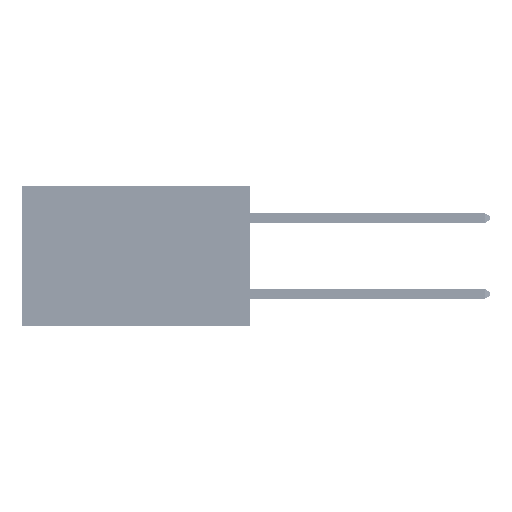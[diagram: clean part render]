
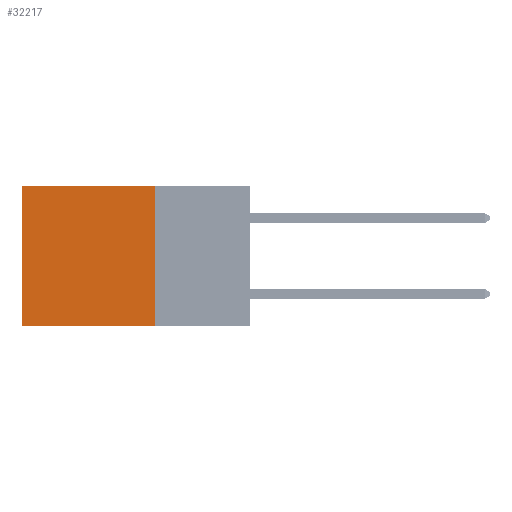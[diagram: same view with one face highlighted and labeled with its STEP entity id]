
A CAD part, left-side view. The second image highlights one B-rep face of the part: STEP entity #32217.
In plain terms, the highlighted planar face has unit normal (-1, 0, 0).
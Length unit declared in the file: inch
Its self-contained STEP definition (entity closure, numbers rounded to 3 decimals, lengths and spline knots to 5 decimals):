
#485 = DIRECTION ( 'NONE',  ( 1., 0., 0. ) ) ;
#1061 = CARTESIAN_POINT ( 'NONE',  ( 0.2875, 0.25, 0. ) ) ;
#2363 = VERTEX_POINT ( 'NONE', #25750 ) ;
#6617 = EDGE_CURVE ( 'NONE', #17309, #47645, #27019, .T. ) ;
#7223 = VECTOR ( 'NONE', #8828, 39.37008 ) ;
#8828 = DIRECTION ( 'NONE',  ( 0., 0., -1. ) ) ;
#8851 = FACE_OUTER_BOUND ( 'NONE', #42961, .T. ) ;
#9224 = CARTESIAN_POINT ( 'NONE',  ( 0.2875, 0.6, 0. ) ) ;
#10294 = ORIENTED_EDGE ( 'NONE', *, *, #19120, .T. ) ;
#11267 = PLANE ( 'NONE',  #15347 ) ;
#12152 = EDGE_CURVE ( 'NONE', #47645, #2363, #40489, .T. ) ;
#15113 = CARTESIAN_POINT ( 'NONE',  ( 0.2875, 0.25, 0. ) ) ;
#15347 = AXIS2_PLACEMENT_3D ( 'NONE', #15113, #485, #38508 ) ;
#17309 = VERTEX_POINT ( 'NONE', #34848 ) ;
#18458 = ORIENTED_EDGE ( 'NONE', *, *, #20578, .T. ) ;
#19120 = EDGE_CURVE ( 'NONE', #31198, #2363, #48873, .T. ) ;
#20578 = EDGE_CURVE ( 'NONE', #17309, #31198, #47485, .T. ) ;
#22829 = VECTOR ( 'NONE', #48923, 39.37008 ) ;
#25750 = CARTESIAN_POINT ( 'NONE',  ( 0.2875, 0.6, -0.37 ) ) ;
#27019 = LINE ( 'NONE', #1061, #7223 ) ;
#27692 = CARTESIAN_POINT ( 'NONE',  ( 0.2875, 0.25, -0.37 ) ) ;
#28824 = ORIENTED_EDGE ( 'NONE', *, *, #12152, .F. ) ;
#31198 = VERTEX_POINT ( 'NONE', #47974 ) ;
#32122 = DIRECTION ( 'NONE',  ( 0., 0., -1. ) ) ;
#32217 = ADVANCED_FACE ( 'NONE', ( #8851 ), #11267, .F. ) ;
#32689 = VECTOR ( 'NONE', #34428, 39.37008 ) ;
#34428 = DIRECTION ( 'NONE',  ( 0., 1., 0. ) ) ;
#34848 = CARTESIAN_POINT ( 'NONE',  ( 0.2875, 0.25, 0. ) ) ;
#37218 = CARTESIAN_POINT ( 'NONE',  ( 0.2875, 0.25, 0. ) ) ;
#38508 = DIRECTION ( 'NONE',  ( 0., 0., -1. ) ) ;
#38699 = VECTOR ( 'NONE', #32122, 39.37008 ) ;
#40489 = LINE ( 'NONE', #46024, #32689 ) ;
#41326 = ORIENTED_EDGE ( 'NONE', *, *, #6617, .F. ) ;
#42961 = EDGE_LOOP ( 'NONE', ( #10294, #28824, #41326, #18458 ) ) ;
#46024 = CARTESIAN_POINT ( 'NONE',  ( 0.2875, 0.25, -0.37 ) ) ;
#47485 = LINE ( 'NONE', #37218, #22829 ) ;
#47645 = VERTEX_POINT ( 'NONE', #27692 ) ;
#47974 = CARTESIAN_POINT ( 'NONE',  ( 0.2875, 0.6, 0. ) ) ;
#48873 = LINE ( 'NONE', #9224, #38699 ) ;
#48923 = DIRECTION ( 'NONE',  ( 0., 1., 0. ) ) ;
